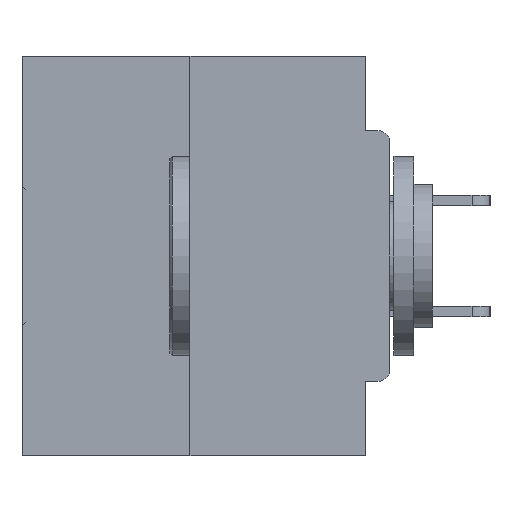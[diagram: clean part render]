
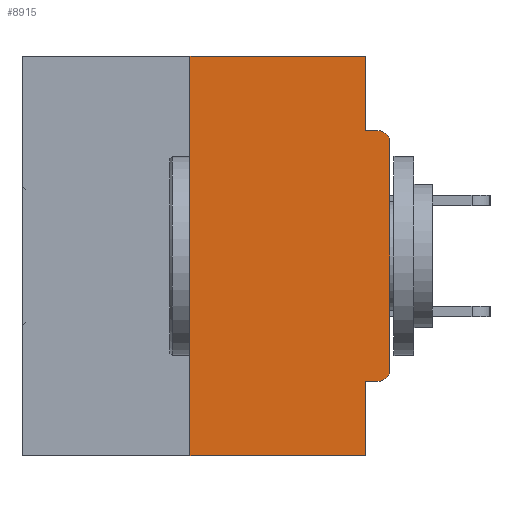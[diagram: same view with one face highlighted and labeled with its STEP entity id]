
A CAD part, left-side view. The second image highlights one B-rep face of the part: STEP entity #8915.
In plain terms, the highlighted planar face has unit normal (-1, 0, 0).
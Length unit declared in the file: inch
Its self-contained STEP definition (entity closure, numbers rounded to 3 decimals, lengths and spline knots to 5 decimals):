
#997 = CARTESIAN_POINT ( 'NONE',  ( 0., 0.015, -0.3915 ) ) ;
#1051 = VERTEX_POINT ( 'NONE', #20598 ) ;
#1616 = VERTEX_POINT ( 'NONE', #38331 ) ;
#1673 = AXIS2_PLACEMENT_3D ( 'NONE', #29690, #16662, #29975 ) ;
#1984 = VECTOR ( 'NONE', #32367, 39.37008 ) ;
#2073 = DIRECTION ( 'NONE',  ( 0., -1., 0. ) ) ;
#2338 = EDGE_CURVE ( 'NONE', #3204, #42376, #9801, .T. ) ;
#2754 = ORIENTED_EDGE ( 'NONE', *, *, #39872, .F. ) ;
#2811 = CARTESIAN_POINT ( 'NONE',  ( 0., 0.031, -0.4065 ) ) ;
#3204 = VERTEX_POINT ( 'NONE', #33288 ) ;
#3309 = DIRECTION ( 'NONE',  ( 0., 0., 1. ) ) ;
#3523 = VECTOR ( 'NONE', #41448, 39.37008 ) ;
#5365 = CARTESIAN_POINT ( 'NONE',  ( 0., 0., -0.4065 ) ) ;
#6588 = ORIENTED_EDGE ( 'NONE', *, *, #32228, .F. ) ;
#6632 = CARTESIAN_POINT ( 'NONE',  ( 0., 0.031, 0. ) ) ;
#7451 = DIRECTION ( 'NONE',  ( 0., 0., -1. ) ) ;
#7899 = PLANE ( 'NONE',  #16120 ) ;
#8159 = LINE ( 'NONE', #9703, #1984 ) ;
#8915 = ADVANCED_FACE ( 'NONE', ( #26746 ), #7899, .F. ) ;
#9551 = CARTESIAN_POINT ( 'NONE',  ( 0., 0.25, 0. ) ) ;
#9703 = CARTESIAN_POINT ( 'NONE',  ( 0., 0., -0.0935 ) ) ;
#9801 = LINE ( 'NONE', #28231, #3523 ) ;
#11115 = CARTESIAN_POINT ( 'NONE',  ( 0., 0.015, -0.0935 ) ) ;
#12310 = DIRECTION ( 'NONE',  ( 0., 1., 0. ) ) ;
#12550 = DIRECTION ( 'NONE',  ( 0., -1., 0. ) ) ;
#13579 = ORIENTED_EDGE ( 'NONE', *, *, #20564, .F. ) ;
#14141 = DIRECTION ( 'NONE',  ( -1., 0., 0. ) ) ;
#14251 = CARTESIAN_POINT ( 'NONE',  ( 0., 0.46, 0. ) ) ;
#14325 = VERTEX_POINT ( 'NONE', #35566 ) ;
#15567 = CARTESIAN_POINT ( 'NONE',  ( 0., 0.031, -0.5 ) ) ;
#15739 = VECTOR ( 'NONE', #3309, 39.37008 ) ;
#16018 = ORIENTED_EDGE ( 'NONE', *, *, #27154, .F. ) ;
#16120 = AXIS2_PLACEMENT_3D ( 'NONE', #14251, #21077, #7451 ) ;
#16662 = DIRECTION ( 'NONE',  ( -1., 0., 0. ) ) ;
#17929 = VERTEX_POINT ( 'NONE', #11115 ) ;
#18015 = ORIENTED_EDGE ( 'NONE', *, *, #32888, .T. ) ;
#18065 = LINE ( 'NONE', #5365, #26244 ) ;
#18249 = EDGE_CURVE ( 'NONE', #30053, #1051, #31289, .T. ) ;
#18475 = CARTESIAN_POINT ( 'NONE',  ( 0., 0.46, -0.5 ) ) ;
#18822 = DIRECTION ( 'NONE',  ( 0., 0., -1. ) ) ;
#19307 = EDGE_LOOP ( 'NONE', ( #6588, #13579, #31099, #26518, #16018, #18015, #36006, #36206, #19763, #2754 ) ) ;
#19369 = CARTESIAN_POINT ( 'NONE',  ( 0., 0.46, 0. ) ) ;
#19763 = ORIENTED_EDGE ( 'NONE', *, *, #33630, .F. ) ;
#20520 = VECTOR ( 'NONE', #2073, 39.37008 ) ;
#20564 = EDGE_CURVE ( 'NONE', #20854, #1616, #27488, .T. ) ;
#20598 = CARTESIAN_POINT ( 'NONE',  ( 0., 0.031, -0.5 ) ) ;
#20854 = VERTEX_POINT ( 'NONE', #39926 ) ;
#21077 = DIRECTION ( 'NONE',  ( 1., 0., 0. ) ) ;
#22133 = LINE ( 'NONE', #19369, #37079 ) ;
#22836 = LINE ( 'NONE', #6632, #33147 ) ;
#25099 = VECTOR ( 'NONE', #18822, 39.37008 ) ;
#25675 = VERTEX_POINT ( 'NONE', #30354 ) ;
#26244 = VECTOR ( 'NONE', #12310, 39.37008 ) ;
#26518 = ORIENTED_EDGE ( 'NONE', *, *, #18249, .F. ) ;
#26746 = FACE_OUTER_BOUND ( 'NONE', #19307, .T. ) ;
#27154 = EDGE_CURVE ( 'NONE', #38336, #30053, #18065, .T. ) ;
#27488 = LINE ( 'NONE', #9551, #15739 ) ;
#27804 = EDGE_CURVE ( 'NONE', #20854, #1051, #36470, .T. ) ;
#28231 = CARTESIAN_POINT ( 'NONE',  ( 0., 0., 0. ) ) ;
#29589 = DIRECTION ( 'NONE',  ( 0., 0., -1. ) ) ;
#29690 = CARTESIAN_POINT ( 'NONE',  ( 0., 0.015, -0.1085 ) ) ;
#29975 = DIRECTION ( 'NONE',  ( 0., 0., -1. ) ) ;
#30050 = CARTESIAN_POINT ( 'NONE',  ( 0., 0.015, -0.4065 ) ) ;
#30053 = VERTEX_POINT ( 'NONE', #2811 ) ;
#30354 = CARTESIAN_POINT ( 'NONE',  ( 0., 0.031, 0. ) ) ;
#30533 = AXIS2_PLACEMENT_3D ( 'NONE', #997, #14141, #37085 ) ;
#31099 = ORIENTED_EDGE ( 'NONE', *, *, #27804, .T. ) ;
#31289 = LINE ( 'NONE', #15567, #25099 ) ;
#32228 = EDGE_CURVE ( 'NONE', #1616, #25675, #22133, .T. ) ;
#32367 = DIRECTION ( 'NONE',  ( 0., -1., 0. ) ) ;
#32888 = EDGE_CURVE ( 'NONE', #38336, #3204, #36994, .T. ) ;
#33147 = VECTOR ( 'NONE', #29589, 39.37008 ) ;
#33199 = EDGE_CURVE ( 'NONE', #42376, #17929, #35417, .T. ) ;
#33288 = CARTESIAN_POINT ( 'NONE',  ( 0., 0., -0.3915 ) ) ;
#33630 = EDGE_CURVE ( 'NONE', #14325, #17929, #8159, .T. ) ;
#35417 = CIRCLE ( 'NONE', #1673, 0.015 ) ;
#35566 = CARTESIAN_POINT ( 'NONE',  ( 0., 0.031, -0.0935 ) ) ;
#36006 = ORIENTED_EDGE ( 'NONE', *, *, #2338, .T. ) ;
#36206 = ORIENTED_EDGE ( 'NONE', *, *, #33199, .T. ) ;
#36470 = LINE ( 'NONE', #18475, #20520 ) ;
#36994 = CIRCLE ( 'NONE', #30533, 0.015 ) ;
#37079 = VECTOR ( 'NONE', #12550, 39.37008 ) ;
#37085 = DIRECTION ( 'NONE',  ( 0., 0., -1. ) ) ;
#38331 = CARTESIAN_POINT ( 'NONE',  ( 0., 0.25, 0. ) ) ;
#38336 = VERTEX_POINT ( 'NONE', #30050 ) ;
#38467 = CARTESIAN_POINT ( 'NONE',  ( 0., 0., -0.1085 ) ) ;
#39872 = EDGE_CURVE ( 'NONE', #25675, #14325, #22836, .T. ) ;
#39926 = CARTESIAN_POINT ( 'NONE',  ( 0., 0.25, -0.5 ) ) ;
#41448 = DIRECTION ( 'NONE',  ( 0., 0., 1. ) ) ;
#42376 = VERTEX_POINT ( 'NONE', #38467 ) ;
